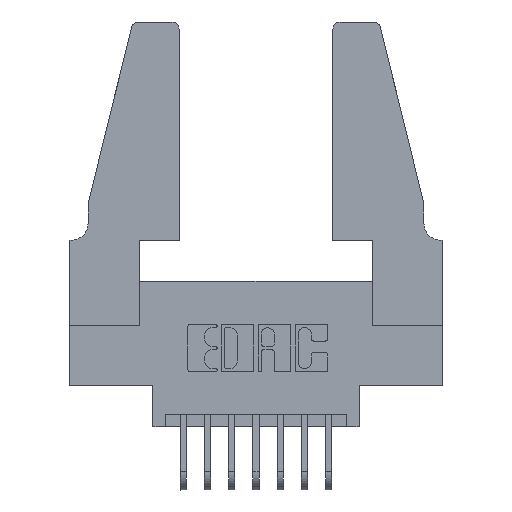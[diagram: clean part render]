
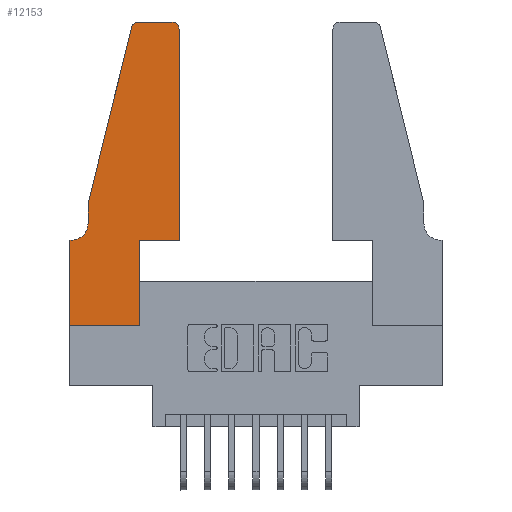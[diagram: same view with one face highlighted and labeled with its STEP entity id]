
A CAD part, top view. The second image highlights one B-rep face of the part: STEP entity #12153.
In plain terms, the highlighted planar face has unit normal (0, 0, 1).
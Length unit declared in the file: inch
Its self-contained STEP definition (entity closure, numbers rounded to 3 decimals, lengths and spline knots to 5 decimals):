
#106 = EDGE_CURVE ( 'NONE', #5108, #3174, #3785, .T. ) ;
#230 = DIRECTION ( 'NONE',  ( 1., 0., 0. ) ) ;
#312 = EDGE_CURVE ( 'NONE', #7438, #1640, #1164, .T. ) ;
#471 = PLANE ( 'NONE',  #1251 ) ;
#741 = AXIS2_PLACEMENT_3D ( 'NONE', #6324, #12019, #7317 ) ;
#1018 = VERTEX_POINT ( 'NONE', #8239 ) ;
#1066 = VECTOR ( 'NONE', #8129, 39.37008 ) ;
#1097 = EDGE_CURVE ( 'NONE', #5651, #7533, #10883, .T. ) ;
#1164 = LINE ( 'NONE', #6467, #1066 ) ;
#1251 = AXIS2_PLACEMENT_3D ( 'NONE', #3049, #9869, #4243 ) ;
#1340 = EDGE_CURVE ( 'NONE', #7533, #9264, #4848, .T. ) ;
#1540 = EDGE_CURVE ( 'NONE', #9264, #1018, #3547, .T. ) ;
#1640 = VERTEX_POINT ( 'NONE', #6798 ) ;
#1755 = VECTOR ( 'NONE', #10953, 39.37008 ) ;
#1765 = EDGE_CURVE ( 'NONE', #1018, #2117, #8249, .T. ) ;
#1935 = EDGE_CURVE ( 'NONE', #2117, #11060, #3154, .T. ) ;
#2117 = VERTEX_POINT ( 'NONE', #4911 ) ;
#2130 = EDGE_CURVE ( 'NONE', #6903, #5651, #6742, .T. ) ;
#2146 = CARTESIAN_POINT ( 'NONE',  ( 0.4505, 0.35, 0.37 ) ) ;
#2474 = VECTOR ( 'NONE', #8355, 39.37008 ) ;
#2563 = ORIENTED_EDGE ( 'NONE', *, *, #2130, .T. ) ;
#2613 = EDGE_CURVE ( 'NONE', #3174, #7438, #3139, .T. ) ;
#2617 = EDGE_CURVE ( 'NONE', #8595, #6903, #3122, .T. ) ;
#2641 = EDGE_CURVE ( 'NONE', #11060, #5108, #2974, .T. ) ;
#2739 = CARTESIAN_POINT ( 'NONE',  ( 0., 0.35, 0.37 ) ) ;
#2885 = ORIENTED_EDGE ( 'NONE', *, *, #2641, .T. ) ;
#2974 = CIRCLE ( 'NONE', #741, 0.03 ) ;
#3049 = CARTESIAN_POINT ( 'NONE',  ( 0., 0.35, 0.37 ) ) ;
#3051 = ORIENTED_EDGE ( 'NONE', *, *, #1097, .T. ) ;
#3122 = CIRCLE ( 'NONE', #11487, 0.07 ) ;
#3139 = CIRCLE ( 'NONE', #9987, 0.03 ) ;
#3154 = LINE ( 'NONE', #2146, #3543 ) ;
#3174 = VERTEX_POINT ( 'NONE', #12047 ) ;
#3543 = VECTOR ( 'NONE', #6613, 39.37008 ) ;
#3547 = LINE ( 'NONE', #11525, #3729 ) ;
#3729 = VECTOR ( 'NONE', #8461, 39.37008 ) ;
#3785 = LINE ( 'NONE', #12341, #2474 ) ;
#3896 = ORIENTED_EDGE ( 'NONE', *, *, #106, .T. ) ;
#3919 = FACE_OUTER_BOUND ( 'NONE', #7638, .T. ) ;
#3951 = CARTESIAN_POINT ( 'NONE',  ( 0.4505, 0.35, 0.37 ) ) ;
#4118 = CARTESIAN_POINT ( 'NONE',  ( 0.0055, 0.42, 0.37 ) ) ;
#4243 = DIRECTION ( 'NONE',  ( 1., 0., 0. ) ) ;
#4257 = ORIENTED_EDGE ( 'NONE', *, *, #2613, .T. ) ;
#4390 = CARTESIAN_POINT ( 'NONE',  ( 0., 0., 0.37 ) ) ;
#4647 = ORIENTED_EDGE ( 'NONE', *, *, #1935, .T. ) ;
#4848 = LINE ( 'NONE', #7134, #5135 ) ;
#4911 = CARTESIAN_POINT ( 'NONE',  ( 0.4505, 0.35, 0.37 ) ) ;
#5108 = VERTEX_POINT ( 'NONE', #7745 ) ;
#5129 = ORIENTED_EDGE ( 'NONE', *, *, #312, .T. ) ;
#5135 = VECTOR ( 'NONE', #230, 39.37008 ) ;
#5216 = DIRECTION ( 'NONE',  ( -1., 0., 0. ) ) ;
#5403 = LINE ( 'NONE', #12242, #1755 ) ;
#5458 = CARTESIAN_POINT ( 'NONE',  ( 0., 0., 0.37 ) ) ;
#5651 = VERTEX_POINT ( 'NONE', #2739 ) ;
#6227 = DIRECTION ( 'NONE',  ( 0., 0., 1. ) ) ;
#6228 = ORIENTED_EDGE ( 'NONE', *, *, #6743, .T. ) ;
#6324 = CARTESIAN_POINT ( 'NONE',  ( 0.4205, 1.22, 0.37 ) ) ;
#6467 = CARTESIAN_POINT ( 'NONE',  ( 0.0755, 0.5, 0.37 ) ) ;
#6613 = DIRECTION ( 'NONE',  ( 0., 1., 0. ) ) ;
#6684 = VECTOR ( 'NONE', #9633, 39.37008 ) ;
#6742 = LINE ( 'NONE', #11172, #6684 ) ;
#6743 = EDGE_CURVE ( 'NONE', #1640, #8595, #5403, .T. ) ;
#6798 = CARTESIAN_POINT ( 'NONE',  ( 0.0755, 0.5, 0.37 ) ) ;
#6820 = CARTESIAN_POINT ( 'NONE',  ( 0.0055, 0.35, 0.37 ) ) ;
#6903 = VERTEX_POINT ( 'NONE', #6820 ) ;
#7134 = CARTESIAN_POINT ( 'NONE',  ( 0., 0., 0.37 ) ) ;
#7212 = ORIENTED_EDGE ( 'NONE', *, *, #1340, .T. ) ;
#7317 = DIRECTION ( 'NONE',  ( 1., 0., 0. ) ) ;
#7320 = ORIENTED_EDGE ( 'NONE', *, *, #1540, .T. ) ;
#7438 = VERTEX_POINT ( 'NONE', #12076 ) ;
#7533 = VERTEX_POINT ( 'NONE', #5458 ) ;
#7638 = EDGE_LOOP ( 'NONE', ( #3896, #4257, #5129, #6228, #9143, #2563, #3051, #7212, #7320, #7678, #4647, #2885 ) ) ;
#7678 = ORIENTED_EDGE ( 'NONE', *, *, #1765, .T. ) ;
#7745 = CARTESIAN_POINT ( 'NONE',  ( 0.4205, 1.25, 0.37 ) ) ;
#8129 = DIRECTION ( 'NONE',  ( -0.239, -0.971, 0. ) ) ;
#8239 = CARTESIAN_POINT ( 'NONE',  ( 0.2865, 0.35, 0.37 ) ) ;
#8249 = LINE ( 'NONE', #3951, #9065 ) ;
#8355 = DIRECTION ( 'NONE',  ( -1., 0., 0. ) ) ;
#8403 = DIRECTION ( 'NONE',  ( 0., -1., 0. ) ) ;
#8461 = DIRECTION ( 'NONE',  ( 0., 1., 0. ) ) ;
#8595 = VERTEX_POINT ( 'NONE', #9241 ) ;
#8812 = CARTESIAN_POINT ( 'NONE',  ( 0.2865, 0., 0.37 ) ) ;
#9065 = VECTOR ( 'NONE', #10476, 39.37008 ) ;
#9143 = ORIENTED_EDGE ( 'NONE', *, *, #2617, .T. ) ;
#9241 = CARTESIAN_POINT ( 'NONE',  ( 0.0755, 0.42, 0.37 ) ) ;
#9264 = VERTEX_POINT ( 'NONE', #8812 ) ;
#9633 = DIRECTION ( 'NONE',  ( -1., 0., 0. ) ) ;
#9754 = CARTESIAN_POINT ( 'NONE',  ( 0.4505, 1.22, 0.37 ) ) ;
#9869 = DIRECTION ( 'NONE',  ( 0., 0., 1. ) ) ;
#9987 = AXIS2_PLACEMENT_3D ( 'NONE', #11297, #6227, #11965 ) ;
#10476 = DIRECTION ( 'NONE',  ( 1., 0., 0. ) ) ;
#10592 = DIRECTION ( 'NONE',  ( 0., 0., -1. ) ) ;
#10650 = VECTOR ( 'NONE', #8403, 39.37008 ) ;
#10883 = LINE ( 'NONE', #4390, #10650 ) ;
#10953 = DIRECTION ( 'NONE',  ( 0., -1., 0. ) ) ;
#11060 = VERTEX_POINT ( 'NONE', #9754 ) ;
#11172 = CARTESIAN_POINT ( 'NONE',  ( 0.0755, 0.35, 0.37 ) ) ;
#11297 = CARTESIAN_POINT ( 'NONE',  ( 0.284, 1.22, 0.37 ) ) ;
#11487 = AXIS2_PLACEMENT_3D ( 'NONE', #4118, #10592, #5216 ) ;
#11525 = CARTESIAN_POINT ( 'NONE',  ( 0.2865, 0.35, 0.37 ) ) ;
#11965 = DIRECTION ( 'NONE',  ( 1., 0., 0. ) ) ;
#12019 = DIRECTION ( 'NONE',  ( 0., 0., 1. ) ) ;
#12047 = CARTESIAN_POINT ( 'NONE',  ( 0.284, 1.25, 0.37 ) ) ;
#12076 = CARTESIAN_POINT ( 'NONE',  ( 0.25487, 1.22718, 0.37 ) ) ;
#12153 = ADVANCED_FACE ( 'NONE', ( #3919 ), #471, .T. ) ;
#12242 = CARTESIAN_POINT ( 'NONE',  ( 0.0755, 0.5, 0.37 ) ) ;
#12341 = CARTESIAN_POINT ( 'NONE',  ( 0.2605, 1.25, 0.37 ) ) ;
